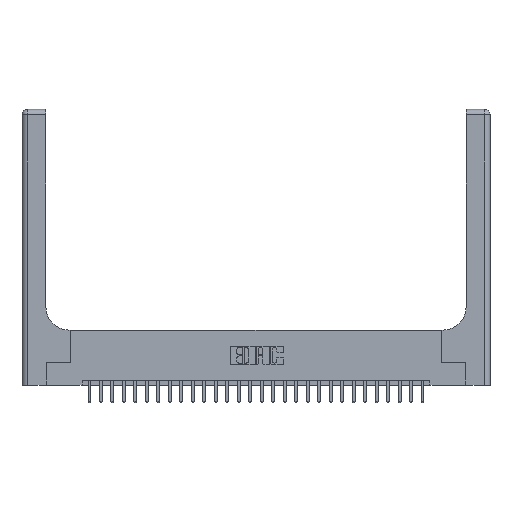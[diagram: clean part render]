
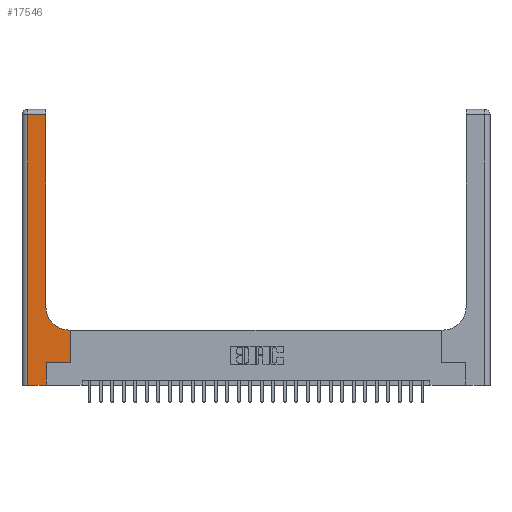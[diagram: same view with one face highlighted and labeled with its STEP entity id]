
A CAD part, top view. The second image highlights one B-rep face of the part: STEP entity #17546.
In plain terms, the highlighted planar face has unit normal (0, 0, 1).
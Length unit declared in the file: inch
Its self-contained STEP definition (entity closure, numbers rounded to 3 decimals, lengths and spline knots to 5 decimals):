
#56 = DIRECTION ( 'NONE',  ( 0., -1., 0. ) ) ;
#150 = CARTESIAN_POINT ( 'NONE',  ( 0.26, 0.6, 0.37 ) ) ;
#161 = DIRECTION ( 'NONE',  ( -1., 0., 0. ) ) ;
#658 = CARTESIAN_POINT ( 'NONE',  ( 0.265, 0., 0.37 ) ) ;
#1088 = EDGE_CURVE ( 'NONE', #19328, #20864, #23416, .T. ) ;
#1437 = ORIENTED_EDGE ( 'NONE', *, *, #8010, .T. ) ;
#2898 = DIRECTION ( 'NONE',  ( 0., 1., 0. ) ) ;
#3416 = VECTOR ( 'NONE', #2898, 39.37008 ) ;
#3948 = CARTESIAN_POINT ( 'NONE',  ( 0., 2.94, 0.37 ) ) ;
#4311 = EDGE_CURVE ( 'NONE', #12630, #7165, #9555, .T. ) ;
#4404 = LINE ( 'NONE', #23387, #15495 ) ;
#4775 = DIRECTION ( 'NONE',  ( 1., 0., 0. ) ) ;
#5181 = DIRECTION ( 'NONE',  ( 0., 0., -1. ) ) ;
#5483 = VERTEX_POINT ( 'NONE', #5618 ) ;
#5618 = CARTESIAN_POINT ( 'NONE',  ( 0.06, 2.94, 0.37 ) ) ;
#5906 = LINE ( 'NONE', #8201, #14882 ) ;
#5999 = LINE ( 'NONE', #3948, #8014 ) ;
#6445 = PLANE ( 'NONE',  #19558 ) ;
#7165 = VERTEX_POINT ( 'NONE', #24164 ) ;
#7173 = VECTOR ( 'NONE', #11658, 39.37008 ) ;
#7500 = VECTOR ( 'NONE', #8416, 39.37008 ) ;
#7931 = ORIENTED_EDGE ( 'NONE', *, *, #1088, .T. ) ;
#8010 = EDGE_CURVE ( 'NONE', #20864, #12630, #13476, .T. ) ;
#8014 = VECTOR ( 'NONE', #161, 39.37008 ) ;
#8201 = CARTESIAN_POINT ( 'NONE',  ( 0., 0., 0.37 ) ) ;
#8319 = DIRECTION ( 'NONE',  ( -1., 0., 0. ) ) ;
#8416 = DIRECTION ( 'NONE',  ( -1., 0., 0. ) ) ;
#9142 = CARTESIAN_POINT ( 'NONE',  ( 0.265, 0.25, 0.37 ) ) ;
#9464 = DIRECTION ( 'NONE',  ( 1., 0., 0. ) ) ;
#9555 = LINE ( 'NONE', #18091, #7173 ) ;
#9584 = ORIENTED_EDGE ( 'NONE', *, *, #13452, .T. ) ;
#9712 = EDGE_LOOP ( 'NONE', ( #15096, #11740, #26531, #20808, #7931, #1437, #19621, #9584, #26218 ) ) ;
#9727 = CARTESIAN_POINT ( 'NONE',  ( 0.265, 0.25, 0.37 ) ) ;
#10152 = VERTEX_POINT ( 'NONE', #15496 ) ;
#10223 = CARTESIAN_POINT ( 'NONE',  ( 0.265, 0., 0.37 ) ) ;
#10255 = FACE_OUTER_BOUND ( 'NONE', #9712, .T. ) ;
#10766 = VECTOR ( 'NONE', #9464, 39.37008 ) ;
#11642 = EDGE_CURVE ( 'NONE', #17234, #5483, #5999, .T. ) ;
#11658 = DIRECTION ( 'NONE',  ( 0., 1., 0. ) ) ;
#11740 = ORIENTED_EDGE ( 'NONE', *, *, #11642, .T. ) ;
#11973 = EDGE_CURVE ( 'NONE', #5483, #19892, #4404, .T. ) ;
#12060 = CARTESIAN_POINT ( 'NONE',  ( 0.06, 0., 0.37 ) ) ;
#12630 = VERTEX_POINT ( 'NONE', #21382 ) ;
#13452 = EDGE_CURVE ( 'NONE', #7165, #18644, #17243, .T. ) ;
#13476 = LINE ( 'NONE', #9727, #10766 ) ;
#14882 = VECTOR ( 'NONE', #24346, 39.37008 ) ;
#15096 = ORIENTED_EDGE ( 'NONE', *, *, #16097, .T. ) ;
#15263 = CARTESIAN_POINT ( 'NONE',  ( 0.51, 0.6, 0.37 ) ) ;
#15495 = VECTOR ( 'NONE', #56, 39.37008 ) ;
#15496 = CARTESIAN_POINT ( 'NONE',  ( 0.26, 0.85, 0.37 ) ) ;
#15758 = LINE ( 'NONE', #22002, #3416 ) ;
#16097 = EDGE_CURVE ( 'NONE', #10152, #17234, #15758, .T. ) ;
#17234 = VERTEX_POINT ( 'NONE', #18795 ) ;
#17243 = LINE ( 'NONE', #150, #7500 ) ;
#17546 = ADVANCED_FACE ( 'NONE', ( #10255 ), #6445, .F. ) ;
#18091 = CARTESIAN_POINT ( 'NONE',  ( 0.528, 0.25, 0.37 ) ) ;
#18644 = VERTEX_POINT ( 'NONE', #15263 ) ;
#18795 = CARTESIAN_POINT ( 'NONE',  ( 0.26, 2.94, 0.37 ) ) ;
#19042 = DIRECTION ( 'NONE',  ( 0., 0., -1. ) ) ;
#19093 = DIRECTION ( 'NONE',  ( 0., 1., 0. ) ) ;
#19153 = VECTOR ( 'NONE', #19093, 39.37008 ) ;
#19328 = VERTEX_POINT ( 'NONE', #10223 ) ;
#19558 = AXIS2_PLACEMENT_3D ( 'NONE', #21216, #19042, #8319 ) ;
#19621 = ORIENTED_EDGE ( 'NONE', *, *, #4311, .T. ) ;
#19892 = VERTEX_POINT ( 'NONE', #12060 ) ;
#19928 = EDGE_CURVE ( 'NONE', #19892, #19328, #5906, .T. ) ;
#20462 = EDGE_CURVE ( 'NONE', #18644, #10152, #21407, .T. ) ;
#20808 = ORIENTED_EDGE ( 'NONE', *, *, #19928, .T. ) ;
#20864 = VERTEX_POINT ( 'NONE', #9142 ) ;
#21216 = CARTESIAN_POINT ( 'NONE',  ( 0., 3., 0.37 ) ) ;
#21382 = CARTESIAN_POINT ( 'NONE',  ( 0.528, 0.25, 0.37 ) ) ;
#21407 = CIRCLE ( 'NONE', #25308, 0.25 ) ;
#22002 = CARTESIAN_POINT ( 'NONE',  ( 0.26, 3., 0.37 ) ) ;
#23387 = CARTESIAN_POINT ( 'NONE',  ( 0.06, 3., 0.37 ) ) ;
#23416 = LINE ( 'NONE', #658, #19153 ) ;
#23876 = CARTESIAN_POINT ( 'NONE',  ( 0.51, 0.85, 0.37 ) ) ;
#24164 = CARTESIAN_POINT ( 'NONE',  ( 0.528, 0.6, 0.37 ) ) ;
#24346 = DIRECTION ( 'NONE',  ( 1., 0., 0. ) ) ;
#25308 = AXIS2_PLACEMENT_3D ( 'NONE', #23876, #5181, #4775 ) ;
#26218 = ORIENTED_EDGE ( 'NONE', *, *, #20462, .T. ) ;
#26531 = ORIENTED_EDGE ( 'NONE', *, *, #11973, .T. ) ;
